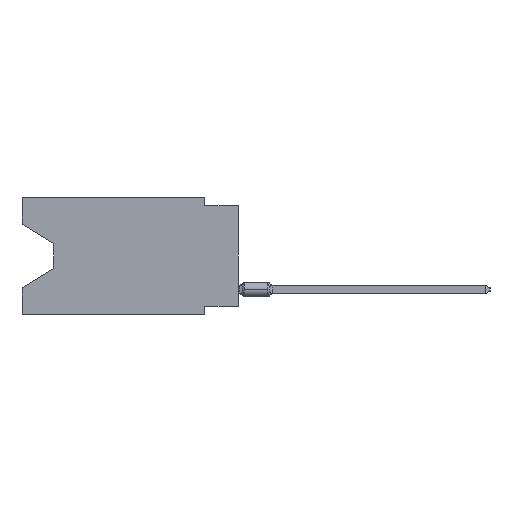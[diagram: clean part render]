
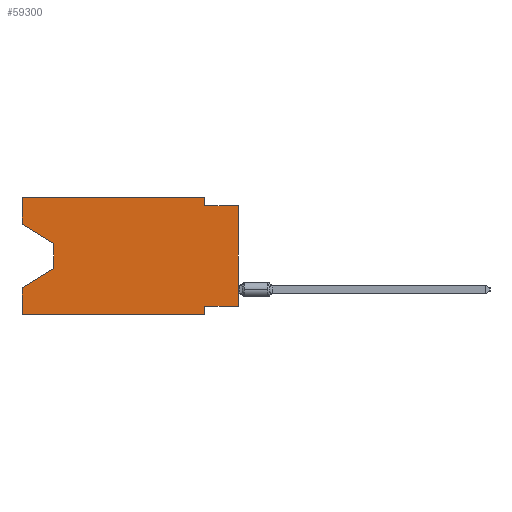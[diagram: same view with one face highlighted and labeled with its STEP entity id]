
A CAD part, left-side view. The second image highlights one B-rep face of the part: STEP entity #59300.
In plain terms, the highlighted planar face has unit normal (-1, 0, 0).
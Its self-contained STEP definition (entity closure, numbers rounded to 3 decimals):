
#1502 = VERTEX_POINT ( 'NONE', #57167 ) ;
#1515 = FACE_OUTER_BOUND ( 'NONE', #81110, .T. ) ;
#2381 = LINE ( 'NONE', #3222, #75269 ) ;
#2485 = ORIENTED_EDGE ( 'NONE', *, *, #25124, .T. ) ;
#2750 = DIRECTION ( 'NONE',  ( 1., 0., 0. ) ) ;
#3222 = CARTESIAN_POINT ( 'NONE',  ( 0., 16.383, 0. ) ) ;
#4648 = VECTOR ( 'NONE', #56510, 1000. ) ;
#6504 = ORIENTED_EDGE ( 'NONE', *, *, #66524, .F. ) ;
#6811 = EDGE_CURVE ( 'NONE', #20370, #81229, #49651, .T. ) ;
#7547 = DIRECTION ( 'NONE',  ( 0., 0., -1. ) ) ;
#8205 = LINE ( 'NONE', #77888, #32634 ) ;
#9179 = LINE ( 'NONE', #15088, #27372 ) ;
#9197 = CARTESIAN_POINT ( 'NONE',  ( 0., 13.97, -5.385 ) ) ;
#9792 = CARTESIAN_POINT ( 'NONE',  ( 0., 16.383, -8.89 ) ) ;
#9793 = EDGE_CURVE ( 'NONE', #18027, #28175, #45117, .T. ) ;
#11877 = CARTESIAN_POINT ( 'NONE',  ( 0., 2.54, -8.89 ) ) ;
#12172 = CARTESIAN_POINT ( 'NONE',  ( 0., 0., -0.635 ) ) ;
#13229 = DIRECTION ( 'NONE',  ( 0., -0.855, -0.519 ) ) ;
#13243 = CARTESIAN_POINT ( 'NONE',  ( 0., 0., -0.635 ) ) ;
#14384 = ORIENTED_EDGE ( 'NONE', *, *, #44491, .F. ) ;
#15088 = CARTESIAN_POINT ( 'NONE',  ( 0., 13.97, -3.505 ) ) ;
#16832 = CARTESIAN_POINT ( 'NONE',  ( 0., 16.383, 0. ) ) ;
#16843 = CARTESIAN_POINT ( 'NONE',  ( 0., 2.54, 0. ) ) ;
#17087 = DIRECTION ( 'NONE',  ( 0., 0., -1. ) ) ;
#18027 = VERTEX_POINT ( 'NONE', #68881 ) ;
#18702 = LINE ( 'NONE', #38396, #39256 ) ;
#18874 = CARTESIAN_POINT ( 'NONE',  ( 0., 0., -8.255 ) ) ;
#19059 = VERTEX_POINT ( 'NONE', #12172 ) ;
#19552 = DIRECTION ( 'NONE',  ( 0., -1., 0. ) ) ;
#20370 = VERTEX_POINT ( 'NONE', #22746 ) ;
#20857 = VECTOR ( 'NONE', #13229, 1000. ) ;
#21692 = DIRECTION ( 'NONE',  ( 0., 0., 1. ) ) ;
#21778 = CARTESIAN_POINT ( 'NONE',  ( 0., 16.383, -6.852 ) ) ;
#22189 = EDGE_CURVE ( 'NONE', #18027, #46761, #37717, .T. ) ;
#22746 = CARTESIAN_POINT ( 'NONE',  ( 0., 2.54, -8.255 ) ) ;
#24730 = CARTESIAN_POINT ( 'NONE',  ( 0., 16.383, 0. ) ) ;
#25124 = EDGE_CURVE ( 'NONE', #1502, #81229, #67286, .T. ) ;
#25140 = DIRECTION ( 'NONE',  ( 0., 0., 1. ) ) ;
#27372 = VECTOR ( 'NONE', #7547, 1000. ) ;
#27931 = DIRECTION ( 'NONE',  ( 0., 0., -1. ) ) ;
#28175 = VERTEX_POINT ( 'NONE', #82107 ) ;
#29785 = VERTEX_POINT ( 'NONE', #82442 ) ;
#31307 = CARTESIAN_POINT ( 'NONE',  ( 0., 13.97, -5.385 ) ) ;
#32634 = VECTOR ( 'NONE', #58573, 1000. ) ;
#33819 = PLANE ( 'NONE',  #38484 ) ;
#34516 = EDGE_CURVE ( 'NONE', #28175, #72637, #9179, .T. ) ;
#35392 = DIRECTION ( 'NONE',  ( 0., -1., 0. ) ) ;
#35859 = EDGE_CURVE ( 'NONE', #72637, #77724, #46976, .T. ) ;
#36367 = EDGE_CURVE ( 'NONE', #60276, #29785, #60711, .T. ) ;
#37717 = LINE ( 'NONE', #24730, #43131 ) ;
#38396 = CARTESIAN_POINT ( 'NONE',  ( 0., 16.383, 0. ) ) ;
#38484 = AXIS2_PLACEMENT_3D ( 'NONE', #79573, #2750, #27931 ) ;
#39256 = VECTOR ( 'NONE', #75384, 1000. ) ;
#39864 = VERTEX_POINT ( 'NONE', #18874 ) ;
#40258 = DIRECTION ( 'NONE',  ( 0., 0.855, -0.519 ) ) ;
#43131 = VECTOR ( 'NONE', #25140, 1000. ) ;
#43147 = VECTOR ( 'NONE', #17087, 1000. ) ;
#44491 = EDGE_CURVE ( 'NONE', #39864, #20370, #55694, .T. ) ;
#45117 = LINE ( 'NONE', #70725, #20857 ) ;
#46761 = VERTEX_POINT ( 'NONE', #16832 ) ;
#46976 = LINE ( 'NONE', #9197, #65049 ) ;
#49651 = LINE ( 'NONE', #11877, #71047 ) ;
#50909 = VECTOR ( 'NONE', #35392, 1000. ) ;
#50914 = EDGE_CURVE ( 'NONE', #1502, #77724, #2381, .T. ) ;
#54344 = CARTESIAN_POINT ( 'NONE',  ( 0., 2.54, -8.89 ) ) ;
#54414 = CARTESIAN_POINT ( 'NONE',  ( 0., 2.54, 0. ) ) ;
#55694 = LINE ( 'NONE', #63215, #4648 ) ;
#56510 = DIRECTION ( 'NONE',  ( 0., 1., 0. ) ) ;
#57167 = CARTESIAN_POINT ( 'NONE',  ( 0., 16.383, -8.89 ) ) ;
#57449 = ORIENTED_EDGE ( 'NONE', *, *, #65484, .F. ) ;
#57681 = ORIENTED_EDGE ( 'NONE', *, *, #34516, .T. ) ;
#58573 = DIRECTION ( 'NONE',  ( 0., 0., 1. ) ) ;
#59300 = ADVANCED_FACE ( 'NONE', ( #1515 ), #33819, .F. ) ;
#60276 = VERTEX_POINT ( 'NONE', #16843 ) ;
#60499 = ORIENTED_EDGE ( 'NONE', *, *, #22189, .F. ) ;
#60711 = LINE ( 'NONE', #54414, #43147 ) ;
#63065 = DIRECTION ( 'NONE',  ( 0., 0., -1. ) ) ;
#63215 = CARTESIAN_POINT ( 'NONE',  ( 0., 0., -8.255 ) ) ;
#64853 = LINE ( 'NONE', #13243, #76673 ) ;
#65049 = VECTOR ( 'NONE', #40258, 1000. ) ;
#65484 = EDGE_CURVE ( 'NONE', #29785, #19059, #64853, .T. ) ;
#66524 = EDGE_CURVE ( 'NONE', #46761, #60276, #18702, .T. ) ;
#66914 = EDGE_CURVE ( 'NONE', #39864, #19059, #8205, .T. ) ;
#67286 = LINE ( 'NONE', #9792, #50909 ) ;
#68375 = ORIENTED_EDGE ( 'NONE', *, *, #6811, .F. ) ;
#68881 = CARTESIAN_POINT ( 'NONE',  ( 0., 16.383, -2.038 ) ) ;
#70725 = CARTESIAN_POINT ( 'NONE',  ( 0., 16.383, -2.038 ) ) ;
#71047 = VECTOR ( 'NONE', #63065, 1000. ) ;
#71378 = ORIENTED_EDGE ( 'NONE', *, *, #50914, .F. ) ;
#72637 = VERTEX_POINT ( 'NONE', #31307 ) ;
#72992 = ORIENTED_EDGE ( 'NONE', *, *, #9793, .T. ) ;
#75269 = VECTOR ( 'NONE', #21692, 1000. ) ;
#75384 = DIRECTION ( 'NONE',  ( 0., -1., 0. ) ) ;
#76673 = VECTOR ( 'NONE', #19552, 1000. ) ;
#77227 = ORIENTED_EDGE ( 'NONE', *, *, #35859, .T. ) ;
#77724 = VERTEX_POINT ( 'NONE', #21778 ) ;
#77888 = CARTESIAN_POINT ( 'NONE',  ( 0., 0., 0. ) ) ;
#78376 = ORIENTED_EDGE ( 'NONE', *, *, #36367, .F. ) ;
#78419 = ORIENTED_EDGE ( 'NONE', *, *, #66914, .T. ) ;
#79573 = CARTESIAN_POINT ( 'NONE',  ( 0., 16.383, 0. ) ) ;
#81110 = EDGE_LOOP ( 'NONE', ( #72992, #57681, #77227, #71378, #2485, #68375, #14384, #78419, #57449, #78376, #6504, #60499 ) ) ;
#81229 = VERTEX_POINT ( 'NONE', #54344 ) ;
#82107 = CARTESIAN_POINT ( 'NONE',  ( 0., 13.97, -3.505 ) ) ;
#82442 = CARTESIAN_POINT ( 'NONE',  ( 0., 2.54, -0.635 ) ) ;
